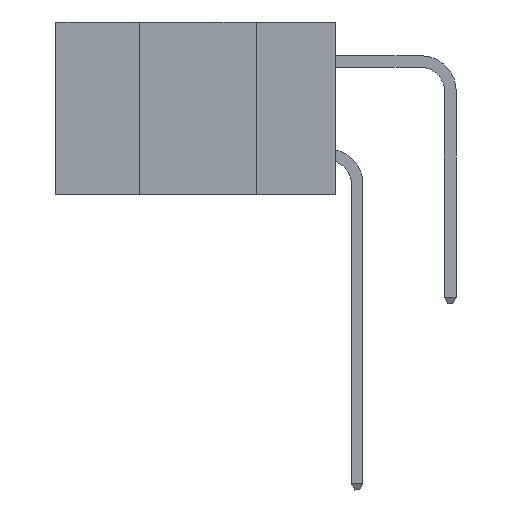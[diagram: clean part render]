
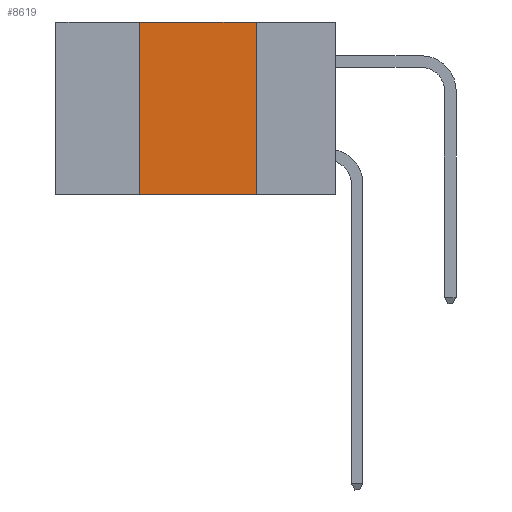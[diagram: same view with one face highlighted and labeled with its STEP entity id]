
A CAD part, left-side view. The second image highlights one B-rep face of the part: STEP entity #8619.
In plain terms, the highlighted planar face has unit normal (-1, 0, 0).
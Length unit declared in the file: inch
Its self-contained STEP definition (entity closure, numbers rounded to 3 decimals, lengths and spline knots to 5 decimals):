
#876 = EDGE_CURVE ( 'NONE', #17535, #8918, #7391, .T. ) ;
#1698 = DIRECTION ( 'NONE',  ( 1., 0., 0. ) ) ;
#2075 = DIRECTION ( 'NONE',  ( 0., -1., 0. ) ) ;
#3684 = CARTESIAN_POINT ( 'NONE',  ( 0., 0.6, 0. ) ) ;
#4330 = DIRECTION ( 'NONE',  ( 0., -1., 0. ) ) ;
#6274 = CARTESIAN_POINT ( 'NONE',  ( 0., 0.6, -0.37 ) ) ;
#6901 = DIRECTION ( 'NONE',  ( 0., 0., -1. ) ) ;
#7391 = LINE ( 'NONE', #20541, #21665 ) ;
#7652 = VECTOR ( 'NONE', #4330, 39.37008 ) ;
#7740 = ORIENTED_EDGE ( 'NONE', *, *, #18123, .T. ) ;
#8619 = ADVANCED_FACE ( 'NONE', ( #11834 ), #19391, .F. ) ;
#8846 = AXIS2_PLACEMENT_3D ( 'NONE', #3684, #1698, #15583 ) ;
#8918 = VERTEX_POINT ( 'NONE', #19027 ) ;
#10358 = CARTESIAN_POINT ( 'NONE',  ( 0., 0.42, 0. ) ) ;
#11035 = CARTESIAN_POINT ( 'NONE',  ( 0., 0.17, 0. ) ) ;
#11528 = LINE ( 'NONE', #17590, #16025 ) ;
#11792 = DIRECTION ( 'NONE',  ( 0., 0., 1. ) ) ;
#11834 = FACE_OUTER_BOUND ( 'NONE', #18806, .T. ) ;
#12521 = LINE ( 'NONE', #21763, #21528 ) ;
#12955 = LINE ( 'NONE', #6274, #7652 ) ;
#13755 = EDGE_CURVE ( 'NONE', #14922, #17535, #12521, .T. ) ;
#13757 = CARTESIAN_POINT ( 'NONE',  ( 0., 0.42, -0.37 ) ) ;
#14922 = VERTEX_POINT ( 'NONE', #10358 ) ;
#15583 = DIRECTION ( 'NONE',  ( 0., 0., -1. ) ) ;
#15988 = EDGE_CURVE ( 'NONE', #22569, #14922, #11528, .T. ) ;
#16025 = VECTOR ( 'NONE', #11792, 39.37008 ) ;
#16888 = ORIENTED_EDGE ( 'NONE', *, *, #876, .F. ) ;
#17535 = VERTEX_POINT ( 'NONE', #11035 ) ;
#17590 = CARTESIAN_POINT ( 'NONE',  ( 0., 0.42, 0. ) ) ;
#18123 = EDGE_CURVE ( 'NONE', #22569, #8918, #12955, .T. ) ;
#18806 = EDGE_LOOP ( 'NONE', ( #16888, #22037, #22627, #7740 ) ) ;
#19027 = CARTESIAN_POINT ( 'NONE',  ( 0., 0.17, -0.37 ) ) ;
#19391 = PLANE ( 'NONE',  #8846 ) ;
#20541 = CARTESIAN_POINT ( 'NONE',  ( 0., 0.17, 0. ) ) ;
#21528 = VECTOR ( 'NONE', #2075, 39.37008 ) ;
#21665 = VECTOR ( 'NONE', #6901, 39.37008 ) ;
#21763 = CARTESIAN_POINT ( 'NONE',  ( 0., 0.6, 0. ) ) ;
#22037 = ORIENTED_EDGE ( 'NONE', *, *, #13755, .F. ) ;
#22569 = VERTEX_POINT ( 'NONE', #13757 ) ;
#22627 = ORIENTED_EDGE ( 'NONE', *, *, #15988, .F. ) ;
